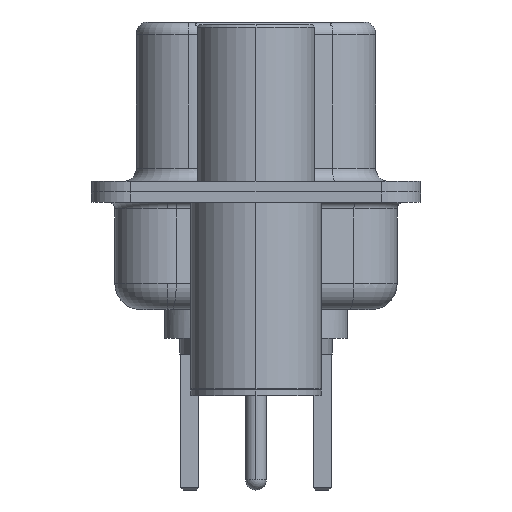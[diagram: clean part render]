
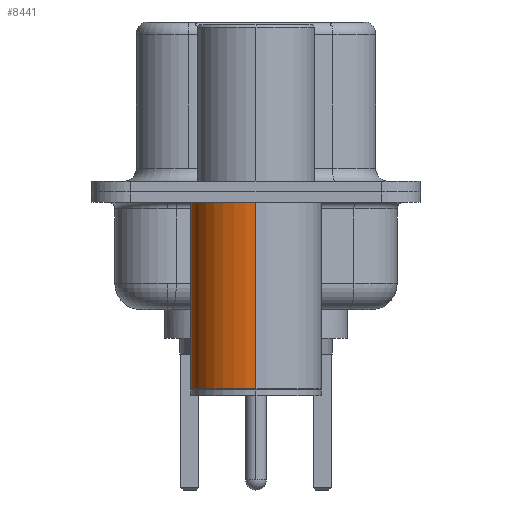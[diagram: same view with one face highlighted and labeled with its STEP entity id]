
A CAD part, left-side view. The second image highlights one B-rep face of the part: STEP entity #8441.
In plain terms, the highlighted cylindrical face has radius 2.5 mm (diameter 5 mm), a partial arc.
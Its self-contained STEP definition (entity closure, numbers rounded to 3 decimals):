
#1459 = DIRECTION ( 'NONE',  ( 1., 0., 0. ) ) ;
#2419 = EDGE_CURVE ( 'NONE', #2989, #3744, #6999, .T. ) ;
#2989 = VERTEX_POINT ( 'NONE', #9847 ) ;
#3099 = CIRCLE ( 'NONE', #12873, 2.5 ) ;
#3123 = DIRECTION ( 'NONE',  ( 0., 0., 1. ) ) ;
#3263 = DIRECTION ( 'NONE',  ( 0., 0., 1. ) ) ;
#3294 = VECTOR ( 'NONE', #11259, 1000. ) ;
#3744 = VERTEX_POINT ( 'NONE', #19427 ) ;
#4109 = DIRECTION ( 'NONE',  ( 1., 0., 0. ) ) ;
#4482 = DIRECTION ( 'NONE',  ( 0., 0., 1. ) ) ;
#4744 = CARTESIAN_POINT ( 'NONE',  ( -2.5, 0., -7.525 ) ) ;
#5172 = EDGE_LOOP ( 'NONE', ( #8341, #15760, #9083, #12251 ) ) ;
#6251 = CARTESIAN_POINT ( 'NONE',  ( 2.5, 0., -7.525 ) ) ;
#6379 = CARTESIAN_POINT ( 'NONE',  ( 0., 0., -0.4 ) ) ;
#6999 = CIRCLE ( 'NONE', #17731, 2.5 ) ;
#7291 = CARTESIAN_POINT ( 'NONE',  ( 0., 0., -7.525 ) ) ;
#8341 = ORIENTED_EDGE ( 'NONE', *, *, #18805, .T. ) ;
#8441 = ADVANCED_FACE ( 'NONE', ( #11812 ), #15053, .T. ) ;
#8916 = VERTEX_POINT ( 'NONE', #6251 ) ;
#9083 = ORIENTED_EDGE ( 'NONE', *, *, #2419, .F. ) ;
#9847 = CARTESIAN_POINT ( 'NONE',  ( 2.5, 0., -0.4 ) ) ;
#10734 = LINE ( 'NONE', #17317, #3294 ) ;
#10823 = CARTESIAN_POINT ( 'NONE',  ( 0., 0., 0.581 ) ) ;
#11048 = AXIS2_PLACEMENT_3D ( 'NONE', #10823, #3123, #20492 ) ;
#11259 = DIRECTION ( 'NONE',  ( 0., 0., 1. ) ) ;
#11676 = EDGE_CURVE ( 'NONE', #15247, #3744, #15453, .T. ) ;
#11791 = EDGE_CURVE ( 'NONE', #8916, #2989, #10734, .T. ) ;
#11812 = FACE_OUTER_BOUND ( 'NONE', #5172, .T. ) ;
#12251 = ORIENTED_EDGE ( 'NONE', *, *, #11791, .F. ) ;
#12873 = AXIS2_PLACEMENT_3D ( 'NONE', #7291, #13613, #4109 ) ;
#13613 = DIRECTION ( 'NONE',  ( 0., 0., 1. ) ) ;
#15053 = CYLINDRICAL_SURFACE ( 'NONE', #11048, 2.5 ) ;
#15247 = VERTEX_POINT ( 'NONE', #4744 ) ;
#15453 = LINE ( 'NONE', #17109, #18965 ) ;
#15760 = ORIENTED_EDGE ( 'NONE', *, *, #11676, .T. ) ;
#17109 = CARTESIAN_POINT ( 'NONE',  ( -2.5, 0., 0.581 ) ) ;
#17317 = CARTESIAN_POINT ( 'NONE',  ( 2.5, 0., 0.581 ) ) ;
#17731 = AXIS2_PLACEMENT_3D ( 'NONE', #6379, #3263, #1459 ) ;
#18805 = EDGE_CURVE ( 'NONE', #8916, #15247, #3099, .T. ) ;
#18965 = VECTOR ( 'NONE', #4482, 1000. ) ;
#19427 = CARTESIAN_POINT ( 'NONE',  ( -2.5, 0., -0.4 ) ) ;
#20492 = DIRECTION ( 'NONE',  ( 1., 0., 0. ) ) ;
